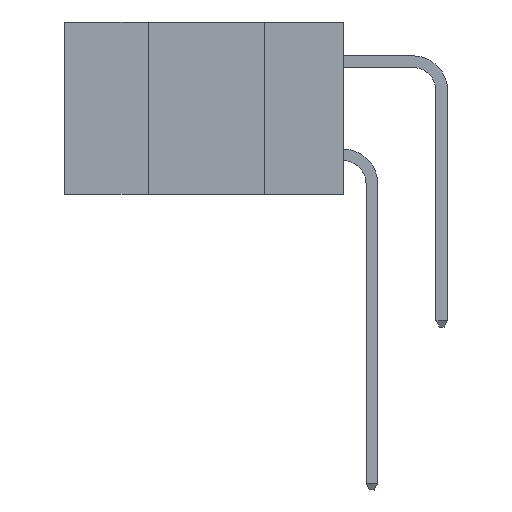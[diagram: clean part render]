
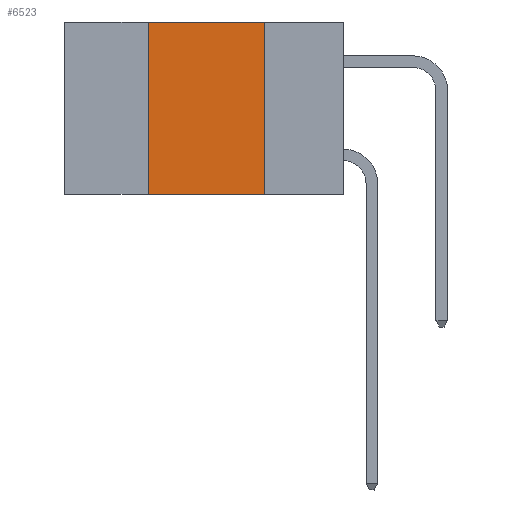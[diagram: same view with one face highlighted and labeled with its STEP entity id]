
A CAD part, left-side view. The second image highlights one B-rep face of the part: STEP entity #6523.
In plain terms, the highlighted planar face has unit normal (-1, 0, 0).
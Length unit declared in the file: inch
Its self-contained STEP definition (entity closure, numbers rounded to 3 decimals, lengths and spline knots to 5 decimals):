
#388 = VECTOR ( 'NONE', #6850, 39.37008 ) ;
#835 = EDGE_LOOP ( 'NONE', ( #13558, #9556, #18625, #5521 ) ) ;
#1214 = VECTOR ( 'NONE', #15530, 39.37008 ) ;
#3328 = CARTESIAN_POINT ( 'NONE',  ( 0., 0.6, -0.37 ) ) ;
#3496 = VECTOR ( 'NONE', #18737, 39.37008 ) ;
#3667 = EDGE_CURVE ( 'NONE', #9352, #17361, #14249, .T. ) ;
#3837 = EDGE_CURVE ( 'NONE', #17361, #6669, #19537, .T. ) ;
#3987 = DIRECTION ( 'NONE',  ( 0., 0., -1. ) ) ;
#4198 = VERTEX_POINT ( 'NONE', #21587 ) ;
#5521 = ORIENTED_EDGE ( 'NONE', *, *, #9359, .T. ) ;
#6523 = ADVANCED_FACE ( 'NONE', ( #20205 ), #21321, .F. ) ;
#6669 = VERTEX_POINT ( 'NONE', #7143 ) ;
#6850 = DIRECTION ( 'NONE',  ( 0., 0., 1. ) ) ;
#6885 = VECTOR ( 'NONE', #3987, 39.37008 ) ;
#7143 = CARTESIAN_POINT ( 'NONE',  ( 0., 0.17, 0. ) ) ;
#7938 = CARTESIAN_POINT ( 'NONE',  ( 0., 0.42, 0. ) ) ;
#8761 = AXIS2_PLACEMENT_3D ( 'NONE', #9452, #12279, #11386 ) ;
#9352 = VERTEX_POINT ( 'NONE', #10259 ) ;
#9359 = EDGE_CURVE ( 'NONE', #9352, #4198, #12157, .T. ) ;
#9452 = CARTESIAN_POINT ( 'NONE',  ( 0., 0.6, 0. ) ) ;
#9556 = ORIENTED_EDGE ( 'NONE', *, *, #3837, .F. ) ;
#10259 = CARTESIAN_POINT ( 'NONE',  ( 0., 0.42, -0.37 ) ) ;
#11386 = DIRECTION ( 'NONE',  ( 0., 0., -1. ) ) ;
#12157 = LINE ( 'NONE', #3328, #3496 ) ;
#12279 = DIRECTION ( 'NONE',  ( 1., 0., 0. ) ) ;
#13558 = ORIENTED_EDGE ( 'NONE', *, *, #13941, .F. ) ;
#13941 = EDGE_CURVE ( 'NONE', #6669, #4198, #15977, .T. ) ;
#14249 = LINE ( 'NONE', #7938, #388 ) ;
#15530 = DIRECTION ( 'NONE',  ( 0., -1., 0. ) ) ;
#15977 = LINE ( 'NONE', #16037, #6885 ) ;
#16037 = CARTESIAN_POINT ( 'NONE',  ( 0., 0.17, 0. ) ) ;
#17361 = VERTEX_POINT ( 'NONE', #19141 ) ;
#18625 = ORIENTED_EDGE ( 'NONE', *, *, #3667, .F. ) ;
#18737 = DIRECTION ( 'NONE',  ( 0., -1., 0. ) ) ;
#19141 = CARTESIAN_POINT ( 'NONE',  ( 0., 0.42, 0. ) ) ;
#19537 = LINE ( 'NONE', #21540, #1214 ) ;
#20205 = FACE_OUTER_BOUND ( 'NONE', #835, .T. ) ;
#21321 = PLANE ( 'NONE',  #8761 ) ;
#21540 = CARTESIAN_POINT ( 'NONE',  ( 0., 0.6, 0. ) ) ;
#21587 = CARTESIAN_POINT ( 'NONE',  ( 0., 0.17, -0.37 ) ) ;
